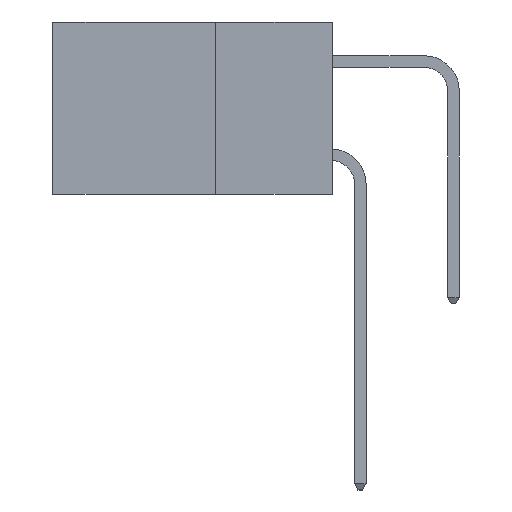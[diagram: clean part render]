
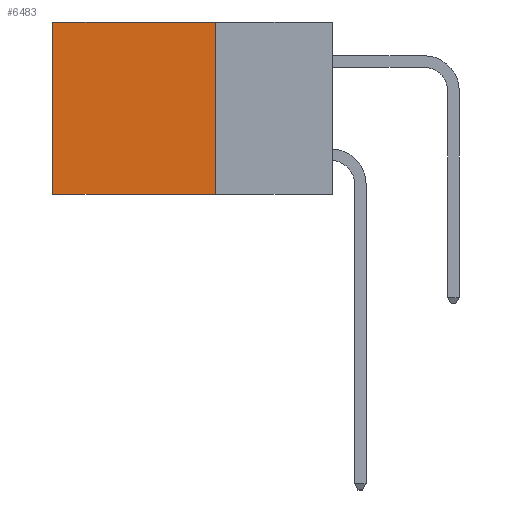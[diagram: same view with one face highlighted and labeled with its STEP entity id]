
A CAD part, left-side view. The second image highlights one B-rep face of the part: STEP entity #6483.
In plain terms, the highlighted planar face has unit normal (-1, 0, 0).
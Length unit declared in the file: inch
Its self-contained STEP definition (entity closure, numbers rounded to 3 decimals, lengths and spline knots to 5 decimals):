
#177 = CARTESIAN_POINT ( 'NONE',  ( 0.2615, 0.25, 0. ) ) ;
#298 = CARTESIAN_POINT ( 'NONE',  ( 0.2615, 0.25, -0.37 ) ) ;
#396 = EDGE_CURVE ( 'NONE', #6293, #6908, #2759, .T. ) ;
#526 = ORIENTED_EDGE ( 'NONE', *, *, #396, .T. ) ;
#803 = VECTOR ( 'NONE', #10719, 39.37008 ) ;
#1417 = FACE_OUTER_BOUND ( 'NONE', #9547, .T. ) ;
#1838 = EDGE_CURVE ( 'NONE', #3073, #6293, #12506, .T. ) ;
#2759 = LINE ( 'NONE', #4887, #13077 ) ;
#3073 = VERTEX_POINT ( 'NONE', #177 ) ;
#3258 = LINE ( 'NONE', #298, #803 ) ;
#3467 = ORIENTED_EDGE ( 'NONE', *, *, #6973, .F. ) ;
#4211 = CARTESIAN_POINT ( 'NONE',  ( 0.2615, 0.25, -0.37 ) ) ;
#4242 = PLANE ( 'NONE',  #5408 ) ;
#4381 = DIRECTION ( 'NONE',  ( 0., 0., -1. ) ) ;
#4887 = CARTESIAN_POINT ( 'NONE',  ( 0.2615, 0.6, -0.37 ) ) ;
#5408 = AXIS2_PLACEMENT_3D ( 'NONE', #11467, #12446, #6376 ) ;
#5468 = ORIENTED_EDGE ( 'NONE', *, *, #9082, .F. ) ;
#6293 = VERTEX_POINT ( 'NONE', #7157 ) ;
#6376 = DIRECTION ( 'NONE',  ( 0., 0., -1. ) ) ;
#6474 = VECTOR ( 'NONE', #10580, 39.37008 ) ;
#6483 = ADVANCED_FACE ( 'NONE', ( #1417 ), #4242, .F. ) ;
#6668 = LINE ( 'NONE', #13197, #12062 ) ;
#6908 = VERTEX_POINT ( 'NONE', #11101 ) ;
#6973 = EDGE_CURVE ( 'NONE', #10166, #6908, #6668, .T. ) ;
#7139 = DIRECTION ( 'NONE',  ( 0., 1., 0. ) ) ;
#7157 = CARTESIAN_POINT ( 'NONE',  ( 0.2615, 0.6, 0. ) ) ;
#8094 = ORIENTED_EDGE ( 'NONE', *, *, #1838, .T. ) ;
#9082 = EDGE_CURVE ( 'NONE', #3073, #10166, #3258, .T. ) ;
#9547 = EDGE_LOOP ( 'NONE', ( #526, #3467, #5468, #8094 ) ) ;
#10166 = VERTEX_POINT ( 'NONE', #4211 ) ;
#10580 = DIRECTION ( 'NONE',  ( 0., 1., 0. ) ) ;
#10719 = DIRECTION ( 'NONE',  ( 0., 0., -1. ) ) ;
#10779 = CARTESIAN_POINT ( 'NONE',  ( 0.2615, 0.25, 0. ) ) ;
#11101 = CARTESIAN_POINT ( 'NONE',  ( 0.2615, 0.6, -0.37 ) ) ;
#11467 = CARTESIAN_POINT ( 'NONE',  ( 0.2615, 0.25, -0.37 ) ) ;
#12062 = VECTOR ( 'NONE', #7139, 39.37008 ) ;
#12446 = DIRECTION ( 'NONE',  ( 1., 0., 0. ) ) ;
#12506 = LINE ( 'NONE', #10779, #6474 ) ;
#13077 = VECTOR ( 'NONE', #4381, 39.37008 ) ;
#13197 = CARTESIAN_POINT ( 'NONE',  ( 0.2615, 0.25, -0.37 ) ) ;
